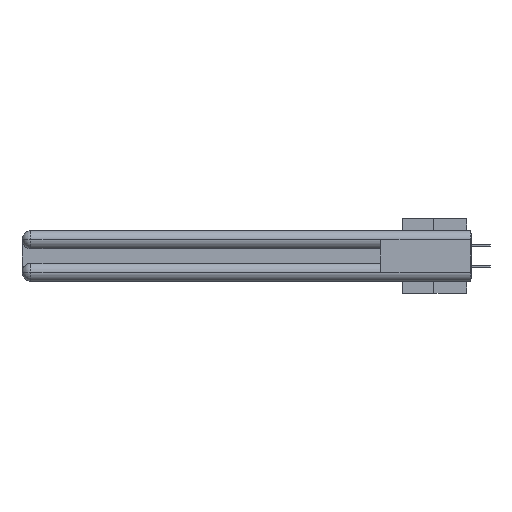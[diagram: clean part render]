
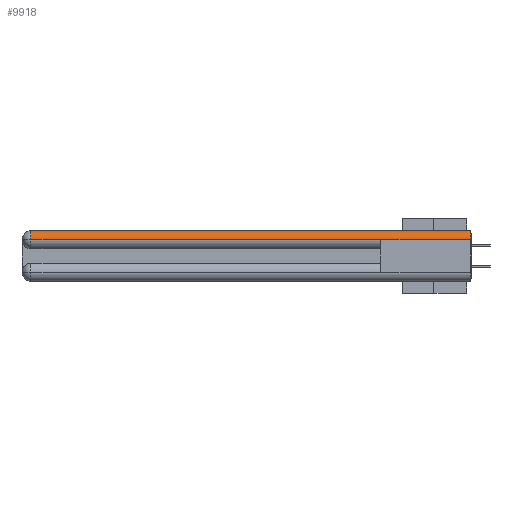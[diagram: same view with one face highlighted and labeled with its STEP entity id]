
A CAD part, left-side view. The second image highlights one B-rep face of the part: STEP entity #9918.
In plain terms, the highlighted cylindrical face has radius 1.562 mm (diameter 3.124 mm), a partial arc.
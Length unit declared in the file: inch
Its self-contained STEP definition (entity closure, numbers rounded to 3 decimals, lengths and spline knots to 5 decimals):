
#370 = DIRECTION ( 'NONE',  ( 0., 1., 0. ) ) ;
#1296 = CYLINDRICAL_SURFACE ( 'NONE', #2075, 0.0615 ) ;
#2052 = VERTEX_POINT ( 'NONE', #33744 ) ;
#2075 = AXIS2_PLACEMENT_3D ( 'NONE', #38500, #370, #25906 ) ;
#6635 = CARTESIAN_POINT ( 'NONE',  ( 0., 0.6, -0.0615 ) ) ;
#8003 = CARTESIAN_POINT ( 'NONE',  ( 0., 2.94, -0.0615 ) ) ;
#8338 = VECTOR ( 'NONE', #13310, 39.37008 ) ;
#9086 = VERTEX_POINT ( 'NONE', #25185 ) ;
#9413 = AXIS2_PLACEMENT_3D ( 'NONE', #39221, #14000, #23711 ) ;
#9740 = FACE_OUTER_BOUND ( 'NONE', #20446, .T. ) ;
#9918 = ADVANCED_FACE ( 'NONE', ( #9740 ), #1296, .T. ) ;
#10598 = DIRECTION ( 'NONE',  ( 0., -1., 0. ) ) ;
#11138 = VERTEX_POINT ( 'NONE', #6635 ) ;
#13310 = DIRECTION ( 'NONE',  ( 0., -1., 0. ) ) ;
#13913 = CIRCLE ( 'NONE', #9413, 0.0615 ) ;
#14000 = DIRECTION ( 'NONE',  ( 0., -1., 0. ) ) ;
#16370 = DIRECTION ( 'NONE',  ( 1., 0., 0. ) ) ;
#16832 = CARTESIAN_POINT ( 'NONE',  ( 0.0615, 0., 0. ) ) ;
#18671 = CIRCLE ( 'NONE', #31324, 0.0615 ) ;
#19125 = ORIENTED_EDGE ( 'NONE', *, *, #26892, .F. ) ;
#19174 = VERTEX_POINT ( 'NONE', #8003 ) ;
#20114 = CARTESIAN_POINT ( 'NONE',  ( 0., 3., -0.0615 ) ) ;
#20251 = EDGE_CURVE ( 'NONE', #9086, #19174, #13913, .T. ) ;
#20446 = EDGE_LOOP ( 'NONE', ( #30330, #33222, #37373, #19125, #33769 ) ) ;
#22035 = EDGE_CURVE ( 'NONE', #35312, #2052, #18671, .T. ) ;
#22330 = CARTESIAN_POINT ( 'NONE',  ( 0., 3., -0.0615 ) ) ;
#22985 = EDGE_CURVE ( 'NONE', #9086, #35312, #23106, .T. ) ;
#23106 = LINE ( 'NONE', #16832, #39104 ) ;
#23309 = DIRECTION ( 'NONE',  ( 0., 1., 0. ) ) ;
#23711 = DIRECTION ( 'NONE',  ( 0., 0., 1. ) ) ;
#24731 = LINE ( 'NONE', #22330, #8338 ) ;
#25185 = CARTESIAN_POINT ( 'NONE',  ( 0.0615, 2.94, 0. ) ) ;
#25906 = DIRECTION ( 'NONE',  ( 0., 0., 1. ) ) ;
#26892 = EDGE_CURVE ( 'NONE', #2052, #11138, #33880, .T. ) ;
#29038 = CARTESIAN_POINT ( 'NONE',  ( 0.0615, 0., -0.0615 ) ) ;
#30330 = ORIENTED_EDGE ( 'NONE', *, *, #22985, .F. ) ;
#30936 = CARTESIAN_POINT ( 'NONE',  ( 0.0615, 0., 0. ) ) ;
#31324 = AXIS2_PLACEMENT_3D ( 'NONE', #29038, #32287, #16370 ) ;
#32287 = DIRECTION ( 'NONE',  ( 0., -1., 0. ) ) ;
#33222 = ORIENTED_EDGE ( 'NONE', *, *, #20251, .T. ) ;
#33744 = CARTESIAN_POINT ( 'NONE',  ( 0., 0., -0.0615 ) ) ;
#33769 = ORIENTED_EDGE ( 'NONE', *, *, #22035, .F. ) ;
#33880 = LINE ( 'NONE', #20114, #38851 ) ;
#35312 = VERTEX_POINT ( 'NONE', #30936 ) ;
#36115 = EDGE_CURVE ( 'NONE', #19174, #11138, #24731, .T. ) ;
#37373 = ORIENTED_EDGE ( 'NONE', *, *, #36115, .T. ) ;
#38500 = CARTESIAN_POINT ( 'NONE',  ( 0.0615, 0., -0.0615 ) ) ;
#38851 = VECTOR ( 'NONE', #23309, 39.37008 ) ;
#39104 = VECTOR ( 'NONE', #10598, 39.37008 ) ;
#39221 = CARTESIAN_POINT ( 'NONE',  ( 0.0615, 2.94, -0.0615 ) ) ;
